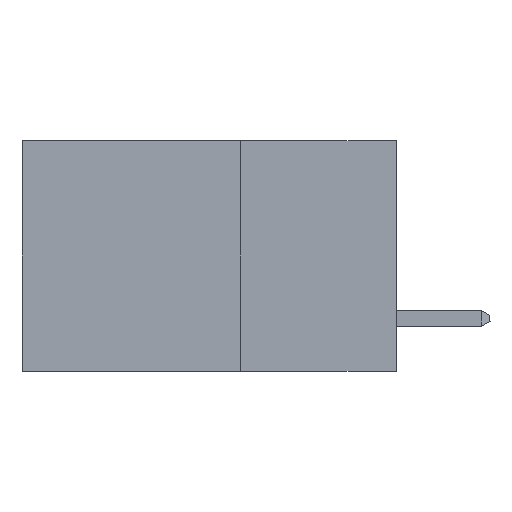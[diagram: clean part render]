
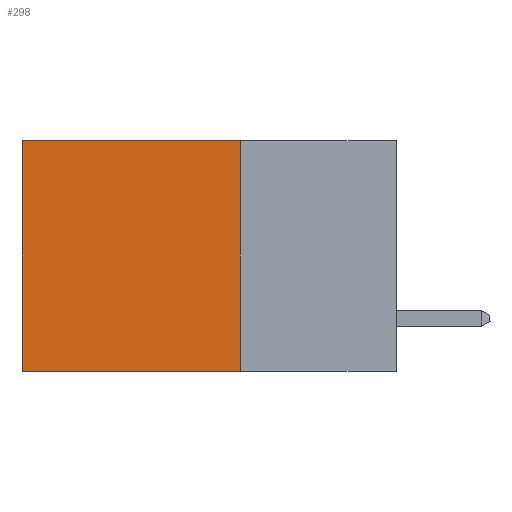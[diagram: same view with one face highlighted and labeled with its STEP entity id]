
A CAD part, left-side view. The second image highlights one B-rep face of the part: STEP entity #298.
In plain terms, the highlighted planar face has unit normal (-1, 0, 0).
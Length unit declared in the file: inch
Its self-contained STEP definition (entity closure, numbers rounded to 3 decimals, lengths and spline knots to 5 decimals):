
#298 = ADVANCED_FACE ( 'NONE', ( #5178 ), #11210, .F. ) ;
#1061 = VECTOR ( 'NONE', #3822, 39.37008 ) ;
#1246 = VECTOR ( 'NONE', #11672, 39.37008 ) ;
#1710 = ORIENTED_EDGE ( 'NONE', *, *, #14652, .F. ) ;
#2365 = LINE ( 'NONE', #11045, #13705 ) ;
#3015 = VECTOR ( 'NONE', #9954, 39.37008 ) ;
#3277 = EDGE_CURVE ( 'NONE', #15769, #14981, #8552, .T. ) ;
#3822 = DIRECTION ( 'NONE',  ( 0., 0., -1. ) ) ;
#4795 = CARTESIAN_POINT ( 'NONE',  ( 0.298, 0.25, 0. ) ) ;
#5031 = VERTEX_POINT ( 'NONE', #16251 ) ;
#5178 = FACE_OUTER_BOUND ( 'NONE', #12688, .T. ) ;
#5993 = LINE ( 'NONE', #16088, #1061 ) ;
#8404 = EDGE_CURVE ( 'NONE', #15214, #5031, #5993, .T. ) ;
#8552 = LINE ( 'NONE', #4795, #1246 ) ;
#9631 = DIRECTION ( 'NONE',  ( 1., 0., 0. ) ) ;
#9822 = DIRECTION ( 'NONE',  ( 0., 0., -1. ) ) ;
#9954 = DIRECTION ( 'NONE',  ( 0., 1., 0. ) ) ;
#10578 = CARTESIAN_POINT ( 'NONE',  ( 0.298, 0.25, -0.37 ) ) ;
#11045 = CARTESIAN_POINT ( 'NONE',  ( 0.298, 0.25, -0.37 ) ) ;
#11210 = PLANE ( 'NONE',  #11776 ) ;
#11672 = DIRECTION ( 'NONE',  ( 0., 0., -1. ) ) ;
#11776 = AXIS2_PLACEMENT_3D ( 'NONE', #12516, #9631, #9822 ) ;
#11851 = CARTESIAN_POINT ( 'NONE',  ( 0.298, 0.6, 0. ) ) ;
#12328 = ORIENTED_EDGE ( 'NONE', *, *, #8404, .T. ) ;
#12516 = CARTESIAN_POINT ( 'NONE',  ( 0.298, 0.25, 0. ) ) ;
#12688 = EDGE_LOOP ( 'NONE', ( #12328, #1710, #12983, #14575 ) ) ;
#12983 = ORIENTED_EDGE ( 'NONE', *, *, #3277, .F. ) ;
#13705 = VECTOR ( 'NONE', #15098, 39.37008 ) ;
#14033 = EDGE_CURVE ( 'NONE', #15769, #15214, #17560, .T. ) ;
#14575 = ORIENTED_EDGE ( 'NONE', *, *, #14033, .T. ) ;
#14652 = EDGE_CURVE ( 'NONE', #14981, #5031, #2365, .T. ) ;
#14929 = CARTESIAN_POINT ( 'NONE',  ( 0.298, 0.25, 0. ) ) ;
#14981 = VERTEX_POINT ( 'NONE', #10578 ) ;
#15098 = DIRECTION ( 'NONE',  ( 0., 1., 0. ) ) ;
#15214 = VERTEX_POINT ( 'NONE', #11851 ) ;
#15769 = VERTEX_POINT ( 'NONE', #14929 ) ;
#16088 = CARTESIAN_POINT ( 'NONE',  ( 0.298, 0.6, 0. ) ) ;
#16251 = CARTESIAN_POINT ( 'NONE',  ( 0.298, 0.6, -0.37 ) ) ;
#16913 = CARTESIAN_POINT ( 'NONE',  ( 0.298, 0.25, 0. ) ) ;
#17560 = LINE ( 'NONE', #16913, #3015 ) ;
